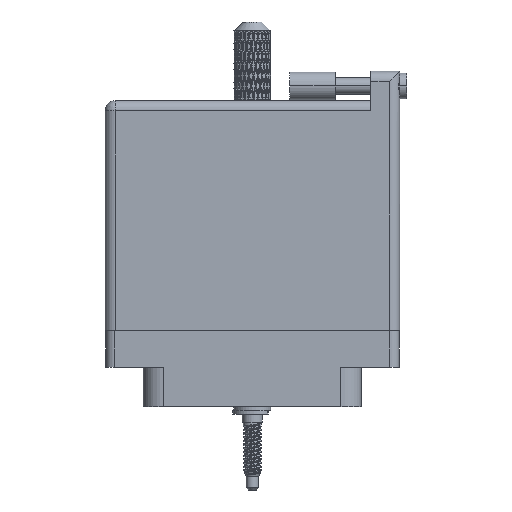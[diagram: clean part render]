
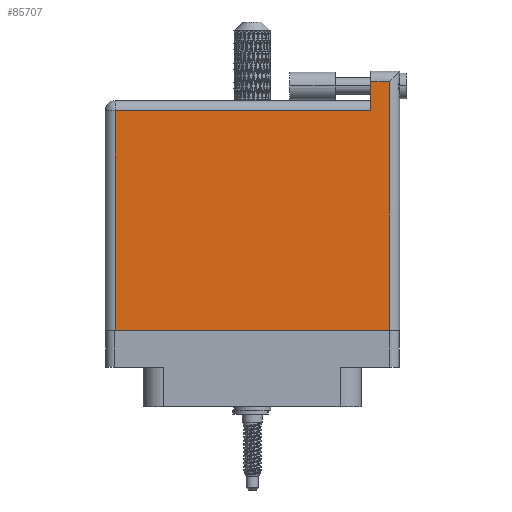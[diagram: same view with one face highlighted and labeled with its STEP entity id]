
A CAD part, front view. The second image highlights one B-rep face of the part: STEP entity #85707.
In plain terms, the highlighted face is planar.
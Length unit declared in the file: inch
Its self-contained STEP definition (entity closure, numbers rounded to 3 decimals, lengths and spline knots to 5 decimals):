
#1635 = ORIENTED_EDGE ( 'NONE', *, *, #80804, .T. ) ;
#3998 = VECTOR ( 'NONE', #17315, 39.37008 ) ;
#5150 = CARTESIAN_POINT ( 'NONE',  ( 0.807, 1.666, 0.4495 ) ) ;
#6529 = AXIS2_PLACEMENT_3D ( 'NONE', #93222, #77123, #85662 ) ;
#10023 = EDGE_CURVE ( 'NONE', #26937, #98813, #14000, .T. ) ;
#10705 = VECTOR ( 'NONE', #39260, 39.37008 ) ;
#12163 = VECTOR ( 'NONE', #33555, 39.37008 ) ;
#13288 = PLANE ( 'NONE',  #6529 ) ;
#14000 = LINE ( 'NONE', #5150, #94994 ) ;
#17315 = DIRECTION ( 'NONE',  ( -1., 0., 0. ) ) ;
#19591 = LINE ( 'NONE', #64653, #12163 ) ;
#23166 = CARTESIAN_POINT ( 'NONE',  ( -1.004, -0.1, 0.4495 ) ) ;
#26937 = VERTEX_POINT ( 'NONE', #70259 ) ;
#27016 = ORIENTED_EDGE ( 'NONE', *, *, #71909, .T. ) ;
#33514 = CARTESIAN_POINT ( 'NONE',  ( -0.934, 1.396, 0.4495 ) ) ;
#33555 = DIRECTION ( 'NONE',  ( 0., -1., 0. ) ) ;
#37079 = CARTESIAN_POINT ( 'NONE',  ( 0.934, 1.596, 0.4495 ) ) ;
#39260 = DIRECTION ( 'NONE',  ( 1., 0., 0. ) ) ;
#41062 = LINE ( 'NONE', #67978, #97456 ) ;
#42515 = EDGE_CURVE ( 'NONE', #98813, #71791, #41062, .T. ) ;
#48173 = CARTESIAN_POINT ( 'NONE',  ( -1.004, 1.596, 0.4495 ) ) ;
#53663 = VERTEX_POINT ( 'NONE', #37079 ) ;
#55361 = VERTEX_POINT ( 'NONE', #70650 ) ;
#59254 = CARTESIAN_POINT ( 'NONE',  ( 0.807, 1.396, 0.4495 ) ) ;
#62759 = ORIENTED_EDGE ( 'NONE', *, *, #79053, .T. ) ;
#63316 = ORIENTED_EDGE ( 'NONE', *, *, #97679, .T. ) ;
#64653 = CARTESIAN_POINT ( 'NONE',  ( -0.934, -0.1, 0.4495 ) ) ;
#66565 = FACE_OUTER_BOUND ( 'NONE', #80751, .T. ) ;
#67978 = CARTESIAN_POINT ( 'NONE',  ( -1.004, 1.396, 0.4495 ) ) ;
#70259 = CARTESIAN_POINT ( 'NONE',  ( 0.807, 1.596, 0.4495 ) ) ;
#70650 = CARTESIAN_POINT ( 'NONE',  ( -0.934, -0.1, 0.4495 ) ) ;
#70847 = LINE ( 'NONE', #23166, #10705 ) ;
#71791 = VERTEX_POINT ( 'NONE', #33514 ) ;
#71909 = EDGE_CURVE ( 'NONE', #55361, #99570, #70847, .T. ) ;
#74148 = VECTOR ( 'NONE', #99296, 39.37008 ) ;
#77123 = DIRECTION ( 'NONE',  ( 0., 0., -1. ) ) ;
#79053 = EDGE_CURVE ( 'NONE', #99570, #53663, #99929, .T. ) ;
#80234 = CARTESIAN_POINT ( 'NONE',  ( 0.934, -0.1, 0.4495 ) ) ;
#80710 = ORIENTED_EDGE ( 'NONE', *, *, #10023, .T. ) ;
#80751 = EDGE_LOOP ( 'NONE', ( #27016, #62759, #1635, #80710, #93800, #63316 ) ) ;
#80804 = EDGE_CURVE ( 'NONE', #53663, #26937, #99842, .T. ) ;
#82096 = DIRECTION ( 'NONE',  ( -1., 0., 0. ) ) ;
#85662 = DIRECTION ( 'NONE',  ( -1., 0., 0. ) ) ;
#85707 = ADVANCED_FACE ( 'NONE', ( #66565 ), #13288, .F. ) ;
#90744 = CARTESIAN_POINT ( 'NONE',  ( 0.934, 1.666, 0.4495 ) ) ;
#93222 = CARTESIAN_POINT ( 'NONE',  ( -1.004, 1.466, 0.4495 ) ) ;
#93800 = ORIENTED_EDGE ( 'NONE', *, *, #42515, .T. ) ;
#94994 = VECTOR ( 'NONE', #97835, 39.37008 ) ;
#97456 = VECTOR ( 'NONE', #82096, 39.37008 ) ;
#97679 = EDGE_CURVE ( 'NONE', #71791, #55361, #19591, .T. ) ;
#97835 = DIRECTION ( 'NONE',  ( 0., -1., 0. ) ) ;
#98813 = VERTEX_POINT ( 'NONE', #59254 ) ;
#99296 = DIRECTION ( 'NONE',  ( 0., 1., 0. ) ) ;
#99570 = VERTEX_POINT ( 'NONE', #80234 ) ;
#99842 = LINE ( 'NONE', #48173, #3998 ) ;
#99929 = LINE ( 'NONE', #90744, #74148 ) ;
